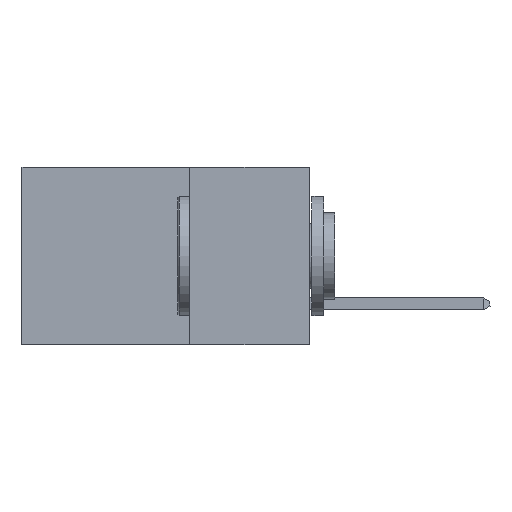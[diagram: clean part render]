
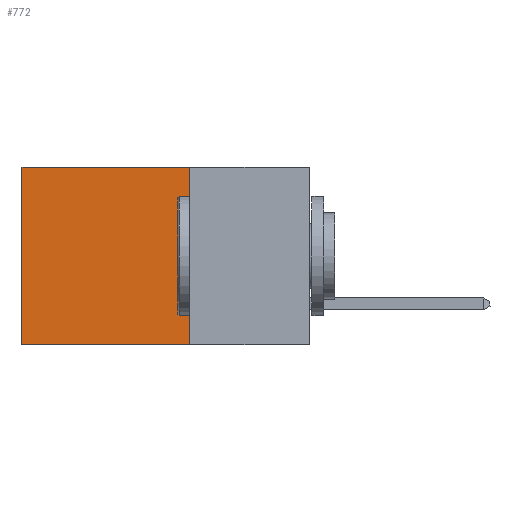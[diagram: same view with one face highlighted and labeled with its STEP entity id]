
A CAD part, left-side view. The second image highlights one B-rep face of the part: STEP entity #772.
In plain terms, the highlighted planar face has unit normal (-1, 0, 0).
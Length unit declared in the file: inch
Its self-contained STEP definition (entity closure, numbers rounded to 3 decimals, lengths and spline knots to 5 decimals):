
#97 = EDGE_CURVE ( 'NONE', #11859, #1614, #5139, .T. ) ;
#158 = EDGE_CURVE ( 'NONE', #1614, #6909, #9412, .T. ) ;
#298 = ORIENTED_EDGE ( 'NONE', *, *, #97, .F. ) ;
#570 = LINE ( 'NONE', #12666, #10184 ) ;
#772 = ADVANCED_FACE ( 'NONE', ( #9039 ), #11771, .F. ) ;
#1076 = DIRECTION ( 'NONE',  ( 0., 1., 0. ) ) ;
#1614 = VERTEX_POINT ( 'NONE', #13392 ) ;
#2408 = DIRECTION ( 'NONE',  ( 0., 0., -1. ) ) ;
#2461 = DIRECTION ( 'NONE',  ( 1., 0., 0. ) ) ;
#3210 = ORIENTED_EDGE ( 'NONE', *, *, #7157, .T. ) ;
#3611 = ORIENTED_EDGE ( 'NONE', *, *, #158, .F. ) ;
#3875 = CARTESIAN_POINT ( 'NONE',  ( 0.2875, 0.25, -0.37 ) ) ;
#5139 = LINE ( 'NONE', #8863, #6582 ) ;
#5947 = CARTESIAN_POINT ( 'NONE',  ( 0.2875, 0.6, 0. ) ) ;
#6582 = VECTOR ( 'NONE', #11677, 39.37008 ) ;
#6909 = VERTEX_POINT ( 'NONE', #9099 ) ;
#7157 = EDGE_CURVE ( 'NONE', #11859, #12736, #570, .T. ) ;
#7911 = EDGE_CURVE ( 'NONE', #12736, #6909, #9356, .T. ) ;
#8405 = DIRECTION ( 'NONE',  ( 0., 0., -1. ) ) ;
#8770 = EDGE_LOOP ( 'NONE', ( #10631, #3611, #298, #3210 ) ) ;
#8863 = CARTESIAN_POINT ( 'NONE',  ( 0.2875, 0.25, 0. ) ) ;
#9039 = FACE_OUTER_BOUND ( 'NONE', #8770, .T. ) ;
#9099 = CARTESIAN_POINT ( 'NONE',  ( 0.2875, 0.6, -0.37 ) ) ;
#9356 = LINE ( 'NONE', #12847, #15844 ) ;
#9412 = LINE ( 'NONE', #3875, #9621 ) ;
#9621 = VECTOR ( 'NONE', #14303, 39.37008 ) ;
#10184 = VECTOR ( 'NONE', #1076, 39.37008 ) ;
#10631 = ORIENTED_EDGE ( 'NONE', *, *, #7911, .T. ) ;
#11677 = DIRECTION ( 'NONE',  ( 0., 0., -1. ) ) ;
#11771 = PLANE ( 'NONE',  #16153 ) ;
#11859 = VERTEX_POINT ( 'NONE', #12056 ) ;
#12056 = CARTESIAN_POINT ( 'NONE',  ( 0.2875, 0.25, 0. ) ) ;
#12666 = CARTESIAN_POINT ( 'NONE',  ( 0.2875, 0.25, 0. ) ) ;
#12736 = VERTEX_POINT ( 'NONE', #5947 ) ;
#12847 = CARTESIAN_POINT ( 'NONE',  ( 0.2875, 0.6, 0. ) ) ;
#13392 = CARTESIAN_POINT ( 'NONE',  ( 0.2875, 0.25, -0.37 ) ) ;
#14303 = DIRECTION ( 'NONE',  ( 0., 1., 0. ) ) ;
#15844 = VECTOR ( 'NONE', #8405, 39.37008 ) ;
#16153 = AXIS2_PLACEMENT_3D ( 'NONE', #16701, #2461, #2408 ) ;
#16701 = CARTESIAN_POINT ( 'NONE',  ( 0.2875, 0.25, 0. ) ) ;
